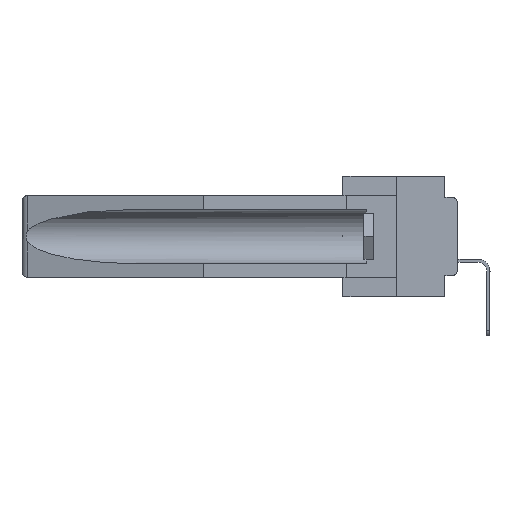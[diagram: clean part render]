
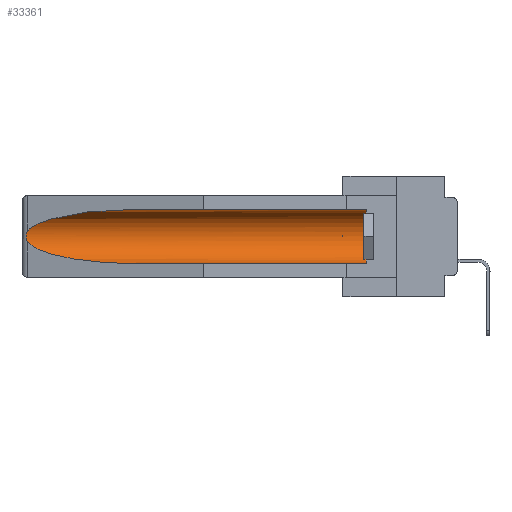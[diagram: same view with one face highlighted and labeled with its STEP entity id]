
A CAD part, left-side view. The second image highlights one B-rep face of the part: STEP entity #33361.
In plain terms, the highlighted cylindrical face has radius 2.857 mm (diameter 5.715 mm), a partial arc.
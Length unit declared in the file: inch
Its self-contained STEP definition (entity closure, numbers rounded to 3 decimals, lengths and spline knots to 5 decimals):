
#2075 = ORIENTED_EDGE ( 'NONE', *, *, #36080, .T. ) ;
#2142 = DIRECTION ( 'NONE',  ( 0., 1., 0. ) ) ;
#3832 = FACE_OUTER_BOUND ( 'NONE', #16750, .T. ) ;
#4042 = VERTEX_POINT ( 'NONE', #30127 ) ;
#4142 = CARTESIAN_POINT ( 'NONE',  ( 0.2673, 1.5327, -0.16383 ) ) ;
#4384 = EDGE_CURVE ( 'NONE', #12623, #31226, #26730, .T. ) ;
#5416 = CARTESIAN_POINT ( 'NONE',  ( 0.26537, 1.52718, -0.19328 ) ) ;
#5562 = CIRCLE ( 'NONE', #9607, 0.1125 ) ;
#6068 = CARTESIAN_POINT ( 'NONE',  ( 0.25451, 1.48313, -0.09465 ) ) ;
#7050 = EDGE_CURVE ( 'NONE', #9073, #4042, #33276, .T. ) ;
#7738 = EDGE_CURVE ( 'NONE', #33911, #8198, #36186, .T. ) ;
#7976 =( BOUNDED_CURVE ( )  B_SPLINE_CURVE ( 3, ( #32097, #20289, #6068, #8931 ),
 .UNSPECIFIED., .F., .F. ) 
 B_SPLINE_CURVE_WITH_KNOTS ( ( 4, 4 ),
 ( 4.71239, 6.08839 ),
 .UNSPECIFIED. ) 
 CURVE ( )  GEOMETRIC_REPRESENTATION_ITEM ( )  RATIONAL_B_SPLINE_CURVE ( ( 1., 0.848, 0.848, 1. ) ) 
 REPRESENTATION_ITEM ( '' )  );
#8198 = VERTEX_POINT ( 'NONE', #30995 ) ;
#8931 = CARTESIAN_POINT ( 'NONE',  ( 0.26537, 1.52718, -0.14972 ) ) ;
#9073 = VERTEX_POINT ( 'NONE', #23253 ) ;
#9607 = AXIS2_PLACEMENT_3D ( 'NONE', #18895, #18767, #27863 ) ;
#9745 = CARTESIAN_POINT ( 'NONE',  ( 0.26597, 1.5296, -0.19026 ) ) ;
#10948 = DIRECTION ( 'NONE',  ( 0., 1., 0. ) ) ;
#11440 = CARTESIAN_POINT ( 'NONE',  ( 0.21114, 1.30732, -0.284 ) ) ;
#12623 = VERTEX_POINT ( 'NONE', #15801 ) ;
#12900 = CARTESIAN_POINT ( 'NONE',  ( 0.26655, 1.53094, -0.18657 ) ) ;
#13027 = CARTESIAN_POINT ( 'NONE',  ( 0.26597, 1.52961, -0.15275 ) ) ;
#13269 = CARTESIAN_POINT ( 'NONE',  ( 0.26537, 1.52718, -0.19328 ) ) ;
#13445 = VECTOR ( 'NONE', #20500, 39.37008 ) ;
#14030 = CARTESIAN_POINT ( 'NONE',  ( 0.155, 1.07973, -0.284 ) ) ;
#15801 = CARTESIAN_POINT ( 'NONE',  ( 0.155, 0.126, -0.059 ) ) ;
#16750 = EDGE_LOOP ( 'NONE', ( #2075, #24985, #29777, #27866, #16931, #26465 ) ) ;
#16931 = ORIENTED_EDGE ( 'NONE', *, *, #38546, .T. ) ;
#17174 = DIRECTION ( 'NONE',  ( 0., 0., 1. ) ) ;
#18767 = DIRECTION ( 'NONE',  ( 0., -1., 0. ) ) ;
#18895 = CARTESIAN_POINT ( 'NONE',  ( 0.155, 0.126, -0.1715 ) ) ;
#19074 = CARTESIAN_POINT ( 'NONE',  ( 0.155, -0.30754, -0.284 ) ) ;
#19780 = EDGE_CURVE ( 'NONE', #4042, #8198, #29221, .T. ) ;
#20289 = CARTESIAN_POINT ( 'NONE',  ( 0.21114, 1.30732, -0.059 ) ) ;
#20500 = DIRECTION ( 'NONE',  ( 0., 1., 0. ) ) ;
#23253 = CARTESIAN_POINT ( 'NONE',  ( 0.26537, 1.52718, -0.14972 ) ) ;
#24831 = CARTESIAN_POINT ( 'NONE',  ( 0.2675, 1.53308, -0.17534 ) ) ;
#24985 = ORIENTED_EDGE ( 'NONE', *, *, #7050, .T. ) ;
#25080 = CARTESIAN_POINT ( 'NONE',  ( 0.26654, 1.53092, -0.15636 ) ) ;
#25586 = CARTESIAN_POINT ( 'NONE',  ( 0.155, 0.126, -0.284 ) ) ;
#25684 = CARTESIAN_POINT ( 'NONE',  ( 0.155, -0.30754, -0.059 ) ) ;
#26465 = ORIENTED_EDGE ( 'NONE', *, *, #4384, .T. ) ;
#26730 = LINE ( 'NONE', #25684, #28601 ) ;
#27581 = CARTESIAN_POINT ( 'NONE',  ( 0.26537, 1.52718, -0.14972 ) ) ;
#27711 = CARTESIAN_POINT ( 'NONE',  ( 0.2673, 1.53269, -0.17917 ) ) ;
#27863 = DIRECTION ( 'NONE',  ( 0., 0., 1. ) ) ;
#27866 = ORIENTED_EDGE ( 'NONE', *, *, #7738, .F. ) ;
#28507 = CYLINDRICAL_SURFACE ( 'NONE', #29311, 0.1125 ) ;
#28601 = VECTOR ( 'NONE', #2142, 39.37008 ) ;
#29221 =( BOUNDED_CURVE ( )  B_SPLINE_CURVE ( 3, ( #5416, #29231, #11440, #14030 ),
 .UNSPECIFIED., .F., .T. ) 
 B_SPLINE_CURVE_WITH_KNOTS ( ( 4, 4 ),
 ( 0.1948, 1.5708 ),
 .UNSPECIFIED. ) 
 CURVE ( )  GEOMETRIC_REPRESENTATION_ITEM ( )  RATIONAL_B_SPLINE_CURVE ( ( 1., 0.848, 0.848, 1. ) ) 
 REPRESENTATION_ITEM ( '' )  );
#29231 = CARTESIAN_POINT ( 'NONE',  ( 0.25451, 1.48313, -0.24835 ) ) ;
#29311 = AXIS2_PLACEMENT_3D ( 'NONE', #31980, #10948, #17174 ) ;
#29777 = ORIENTED_EDGE ( 'NONE', *, *, #19780, .T. ) ;
#30127 = CARTESIAN_POINT ( 'NONE',  ( 0.26537, 1.52718, -0.19328 ) ) ;
#30995 = CARTESIAN_POINT ( 'NONE',  ( 0.155, 1.07973, -0.284 ) ) ;
#31073 = CARTESIAN_POINT ( 'NONE',  ( 0.2675, 1.53308, -0.16763 ) ) ;
#31226 = VERTEX_POINT ( 'NONE', #33663 ) ;
#31980 = CARTESIAN_POINT ( 'NONE',  ( 0.155, -0.30754, -0.1715 ) ) ;
#32097 = CARTESIAN_POINT ( 'NONE',  ( 0.155, 1.07973, -0.059 ) ) ;
#33276 = B_SPLINE_CURVE_WITH_KNOTS ( 'NONE', 3,
 ( #27581, #13027, #25080, #4142, #31073, #24831, #27711, #12900, #9745, #13269 ),
 .UNSPECIFIED., .F., .F.,
 ( 4, 2, 2, 2, 4 ),
 ( 0., 0.00029, 0.00058, 0.00087, 0.00117 ),
 .UNSPECIFIED. ) ;
#33361 = ADVANCED_FACE ( 'NONE', ( #3832 ), #28507, .F. ) ;
#33663 = CARTESIAN_POINT ( 'NONE',  ( 0.155, 1.07973, -0.059 ) ) ;
#33911 = VERTEX_POINT ( 'NONE', #25586 ) ;
#36080 = EDGE_CURVE ( 'NONE', #31226, #9073, #7976, .T. ) ;
#36186 = LINE ( 'NONE', #19074, #13445 ) ;
#38546 = EDGE_CURVE ( 'NONE', #33911, #12623, #5562, .T. ) ;
